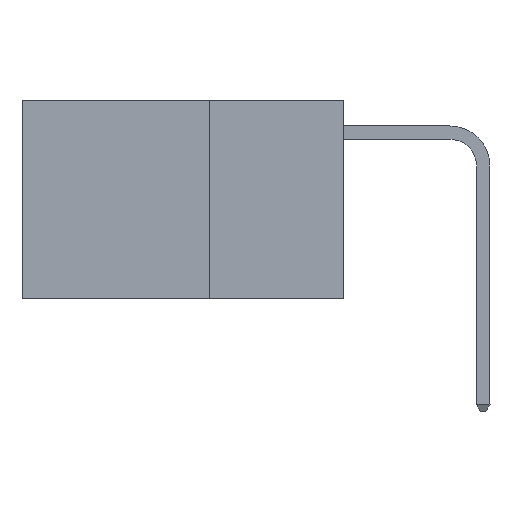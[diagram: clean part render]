
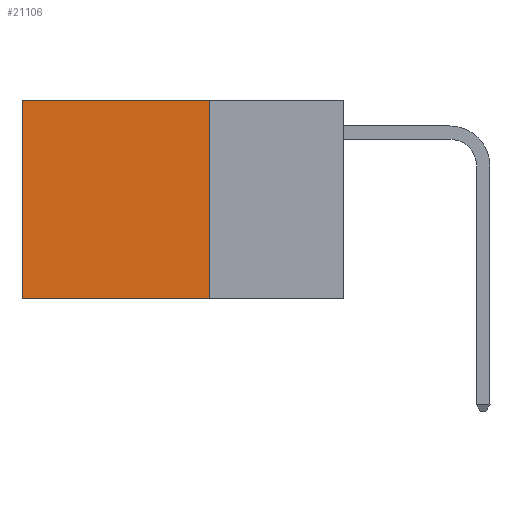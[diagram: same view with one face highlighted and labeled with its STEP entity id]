
A CAD part, left-side view. The second image highlights one B-rep face of the part: STEP entity #21106.
In plain terms, the highlighted planar face has unit normal (-1, 0, 0).
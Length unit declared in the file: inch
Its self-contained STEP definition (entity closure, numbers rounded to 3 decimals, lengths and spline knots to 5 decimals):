
#1408 = ORIENTED_EDGE ( 'NONE', *, *, #2258, .T. ) ;
#1814 = EDGE_CURVE ( 'NONE', #24505, #25339, #24573, .T. ) ;
#1941 = CARTESIAN_POINT ( 'NONE',  ( 0.2625, 0.6, 0. ) ) ;
#2258 = EDGE_CURVE ( 'NONE', #16249, #25339, #10425, .T. ) ;
#2644 = ORIENTED_EDGE ( 'NONE', *, *, #1814, .F. ) ;
#3391 = VECTOR ( 'NONE', #17701, 39.37008 ) ;
#3700 = LINE ( 'NONE', #9511, #3391 ) ;
#3810 = CARTESIAN_POINT ( 'NONE',  ( 0.2625, 0.25, -0.37 ) ) ;
#5063 = ORIENTED_EDGE ( 'NONE', *, *, #23007, .T. ) ;
#5698 = FACE_OUTER_BOUND ( 'NONE', #19847, .T. ) ;
#9511 = CARTESIAN_POINT ( 'NONE',  ( 0.2625, 0.25, 0. ) ) ;
#10321 = DIRECTION ( 'NONE',  ( 0., 1., 0. ) ) ;
#10408 = DIRECTION ( 'NONE',  ( 0., 1., 0. ) ) ;
#10425 = LINE ( 'NONE', #1941, #21070 ) ;
#11821 = VECTOR ( 'NONE', #10408, 39.37008 ) ;
#12234 = CARTESIAN_POINT ( 'NONE',  ( 0.2625, 0.6, 0. ) ) ;
#12435 = CARTESIAN_POINT ( 'NONE',  ( 0.2625, 0.25, 0. ) ) ;
#12780 = CARTESIAN_POINT ( 'NONE',  ( 0.2625, 0.25, 0. ) ) ;
#12809 = EDGE_CURVE ( 'NONE', #15801, #24505, #3700, .T. ) ;
#13027 = AXIS2_PLACEMENT_3D ( 'NONE', #19575, #23614, #17425 ) ;
#14751 = CARTESIAN_POINT ( 'NONE',  ( 0.2625, 0.25, -0.37 ) ) ;
#15223 = CARTESIAN_POINT ( 'NONE',  ( 0.2625, 0.6, -0.37 ) ) ;
#15801 = VERTEX_POINT ( 'NONE', #12780 ) ;
#16249 = VERTEX_POINT ( 'NONE', #12234 ) ;
#16732 = DIRECTION ( 'NONE',  ( 0., 0., -1. ) ) ;
#17113 = ORIENTED_EDGE ( 'NONE', *, *, #12809, .F. ) ;
#17425 = DIRECTION ( 'NONE',  ( 0., 0., -1. ) ) ;
#17701 = DIRECTION ( 'NONE',  ( 0., 0., -1. ) ) ;
#19575 = CARTESIAN_POINT ( 'NONE',  ( 0.2625, 0.25, 0. ) ) ;
#19847 = EDGE_LOOP ( 'NONE', ( #1408, #2644, #17113, #5063 ) ) ;
#21070 = VECTOR ( 'NONE', #16732, 39.37008 ) ;
#21106 = ADVANCED_FACE ( 'NONE', ( #5698 ), #26167, .F. ) ;
#22374 = VECTOR ( 'NONE', #10321, 39.37008 ) ;
#23007 = EDGE_CURVE ( 'NONE', #15801, #16249, #24258, .T. ) ;
#23614 = DIRECTION ( 'NONE',  ( 1., 0., 0. ) ) ;
#24258 = LINE ( 'NONE', #12435, #11821 ) ;
#24505 = VERTEX_POINT ( 'NONE', #3810 ) ;
#24573 = LINE ( 'NONE', #14751, #22374 ) ;
#25339 = VERTEX_POINT ( 'NONE', #15223 ) ;
#26167 = PLANE ( 'NONE',  #13027 ) ;
